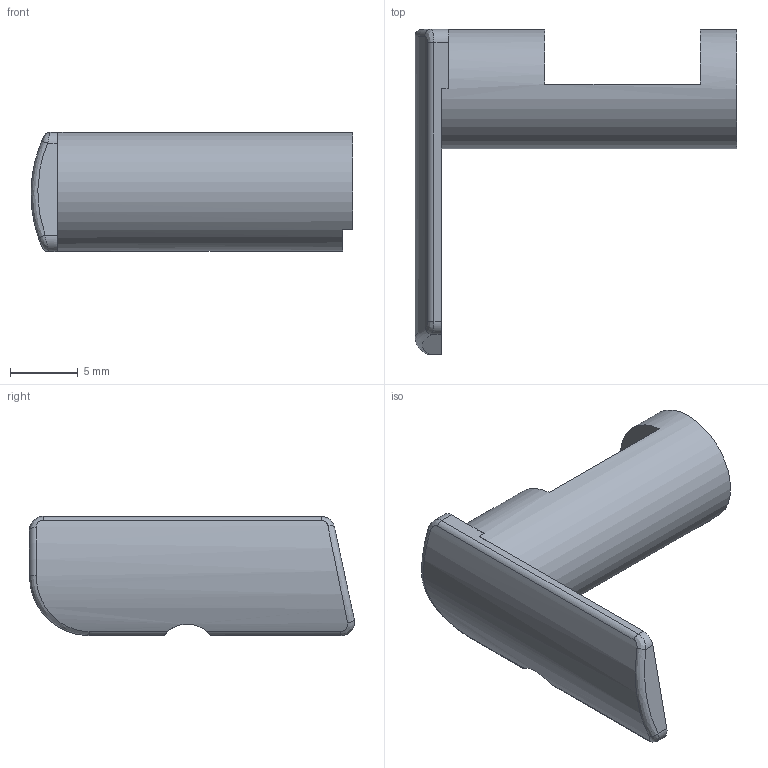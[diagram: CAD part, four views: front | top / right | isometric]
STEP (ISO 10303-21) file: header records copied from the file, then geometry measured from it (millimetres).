
FILE_DESCRIPTION(/* description */ (''),/* implementation_level */ '2;1');
FILE_NAME(/* name */ 'Disassembly Lug.step',/* time_stamp */ '2021-03-06T17:01:35-05:00',/* author */ (''),/* organization */ (''),/* preprocessor_version */ 'ST-DEVELOPER v18.1',/* originating_system */ 'Autodesk Translation Framework v9.10.0.1330',/* authorisation */ '');
FILE_SCHEMA (('AUTOMOTIVE_DESIGN { 1 0 10303 214 3 1 1 }'));
Length unit declared in the file: millimetre
Products named in the file (1): Disassembly Lug
Bounding box: 23.79 x 24.01 x 8.8 mm (x, y, z)
Volume: 1329.8 mm3; surface area: 1075.7 mm2
Topology: 1 solids, 1 shells, 28 faces, 67 edges, 42 vertices
Faces by surface type: plane 13, cylinder 9, bspline 5, torus 1
Full cylindrical faces by diameter (mm): 8.8 x1
Entity records: 1010 total; most frequent: CARTESIAN_POINT 334, ORIENTED_EDGE 134, DIRECTION 128, EDGE_CURVE 67, AXIS2_PLACEMENT_3D 48, VERTEX_POINT 42, LINE 32, VECTOR 32
